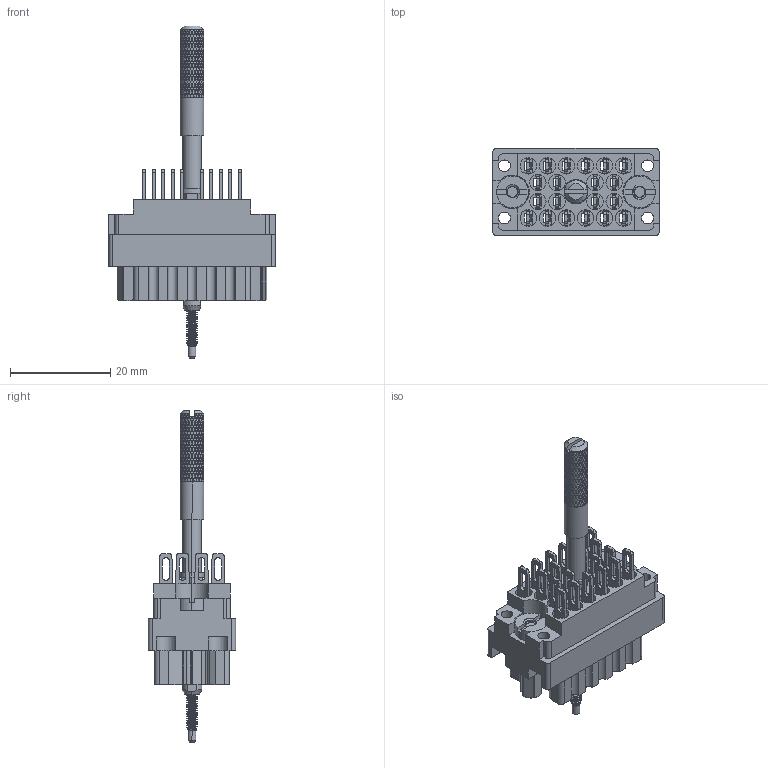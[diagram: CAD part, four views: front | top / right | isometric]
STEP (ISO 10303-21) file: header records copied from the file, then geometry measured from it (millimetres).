
FILE_DESCRIPTION (( 'STEP AP203' ), '1' );
FILE_NAME ('516-020-500-401.STEP', '2020-03-04T17:43:32', ( '' ), ( '' ), 'SwSTEP 2.0', 'SolidWorks 2016', '' );
FILE_SCHEMA (( 'CONFIG_CONTROL_DESIGN' ));
Length unit declared in the file: inch
Products named in the file (12): 516-221-020-102_021; 516-250-021-102; 516-252-021-102_020; 516-250-020-111; 516 Part Receptacle_020; 516-253-025-100; 516-221-020-102_020; Actuating Screw Assy 020; 516-251-025-100; 516-252-022-102; 516-292-001_500 Contact; 516-020-500-401
Assembly tree (31 placements, depth 3):
  516-020-500-401
    516 Part Receptacle_020
    516-292-001_500 Contact  x20
    516-252-021-102_020  x2
    516-221-020-102_020
    Actuating Screw Assy 020
      516-251-025-100
      516-250-021-102
      516-250-020-111
      516-253-025-100
      516-252-022-102
    516-221-020-102_021
Bounding box: 33.32 x 17.42 x 66.29 mm (x, y, z)
Volume: 6863.8 mm3; surface area: 14061.8 mm2
Topology: 30 solids, 30 shells, 4981 faces, 12220 edges, 7310 vertices
Faces by surface type: bspline 2170, plane 1398, cylinder 1357, cone 56
Entity records: 191194 total; most frequent: CARTESIAN_POINT 134579, ORIENTED_EDGE 15892, EDGE_CURVE 7946, DIRECTION 6186, VERTEX_POINT 4476, EDGE_LOOP 3590, ADVANCED_FACE 3506, FACE_OUTER_BOUND 3506
